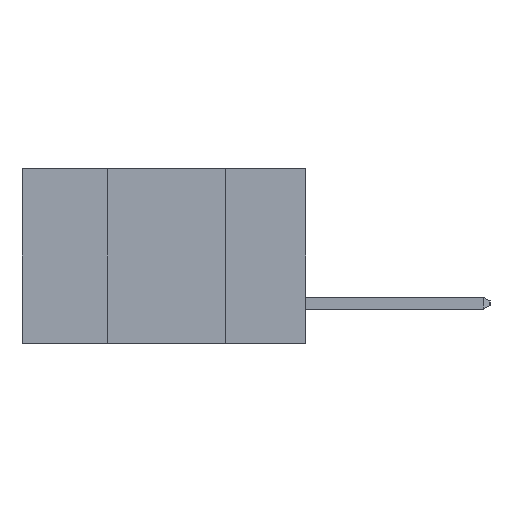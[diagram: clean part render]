
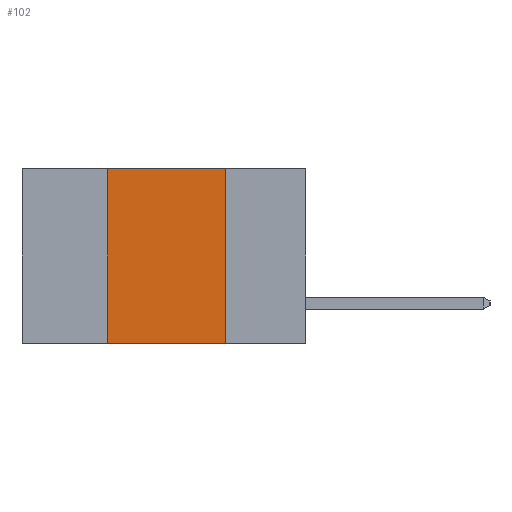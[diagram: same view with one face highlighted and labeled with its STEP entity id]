
A CAD part, left-side view. The second image highlights one B-rep face of the part: STEP entity #102.
In plain terms, the highlighted planar face has unit normal (-1, 0, 0).
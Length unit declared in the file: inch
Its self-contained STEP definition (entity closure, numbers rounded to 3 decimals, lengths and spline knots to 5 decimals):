
#102 = ADVANCED_FACE ( 'NONE', ( #9268 ), #6424, .F. ) ;
#322 = ORIENTED_EDGE ( 'NONE', *, *, #838, .F. ) ;
#335 = VERTEX_POINT ( 'NONE', #578 ) ;
#578 = CARTESIAN_POINT ( 'NONE',  ( 0., 0.17, 0. ) ) ;
#655 = DIRECTION ( 'NONE',  ( 0., 0., -1. ) ) ;
#838 = EDGE_CURVE ( 'NONE', #335, #3721, #6079, .T. ) ;
#1370 = EDGE_CURVE ( 'NONE', #3884, #3721, #1635, .T. ) ;
#1635 = LINE ( 'NONE', #8135, #9436 ) ;
#2396 = CARTESIAN_POINT ( 'NONE',  ( 0., 0.42, -0.37 ) ) ;
#2499 = EDGE_LOOP ( 'NONE', ( #322, #2789, #8969, #5194 ) ) ;
#2789 = ORIENTED_EDGE ( 'NONE', *, *, #8278, .F. ) ;
#2905 = CARTESIAN_POINT ( 'NONE',  ( 0., 0.42, -0.37 ) ) ;
#3283 = DIRECTION ( 'NONE',  ( 1., 0., 0. ) ) ;
#3396 = LINE ( 'NONE', #7632, #7381 ) ;
#3721 = VERTEX_POINT ( 'NONE', #8981 ) ;
#3792 = CARTESIAN_POINT ( 'NONE',  ( 0., 0.17, -0.37 ) ) ;
#3884 = VERTEX_POINT ( 'NONE', #2396 ) ;
#3919 = DIRECTION ( 'NONE',  ( 0., -1., 0. ) ) ;
#4827 = VECTOR ( 'NONE', #8831, 39.37008 ) ;
#5076 = EDGE_CURVE ( 'NONE', #3884, #5309, #8700, .T. ) ;
#5194 = ORIENTED_EDGE ( 'NONE', *, *, #1370, .T. ) ;
#5309 = VERTEX_POINT ( 'NONE', #6164 ) ;
#5591 = VECTOR ( 'NONE', #5953, 39.37008 ) ;
#5907 = CARTESIAN_POINT ( 'NONE',  ( 0., 0.6, 0. ) ) ;
#5953 = DIRECTION ( 'NONE',  ( 0., 0., -1. ) ) ;
#6079 = LINE ( 'NONE', #3792, #5591 ) ;
#6164 = CARTESIAN_POINT ( 'NONE',  ( 0., 0.42, 0. ) ) ;
#6424 = PLANE ( 'NONE',  #6951 ) ;
#6951 = AXIS2_PLACEMENT_3D ( 'NONE', #5907, #3283, #655 ) ;
#7381 = VECTOR ( 'NONE', #3919, 39.37008 ) ;
#7632 = CARTESIAN_POINT ( 'NONE',  ( 0., 0.6, 0. ) ) ;
#8135 = CARTESIAN_POINT ( 'NONE',  ( 0., 0.6, -0.37 ) ) ;
#8278 = EDGE_CURVE ( 'NONE', #5309, #335, #3396, .T. ) ;
#8700 = LINE ( 'NONE', #2905, #4827 ) ;
#8831 = DIRECTION ( 'NONE',  ( 0., 0., 1. ) ) ;
#8969 = ORIENTED_EDGE ( 'NONE', *, *, #5076, .F. ) ;
#8981 = CARTESIAN_POINT ( 'NONE',  ( 0., 0.17, -0.37 ) ) ;
#9268 = FACE_OUTER_BOUND ( 'NONE', #2499, .T. ) ;
#9436 = VECTOR ( 'NONE', #9908, 39.37008 ) ;
#9908 = DIRECTION ( 'NONE',  ( 0., -1., 0. ) ) ;
